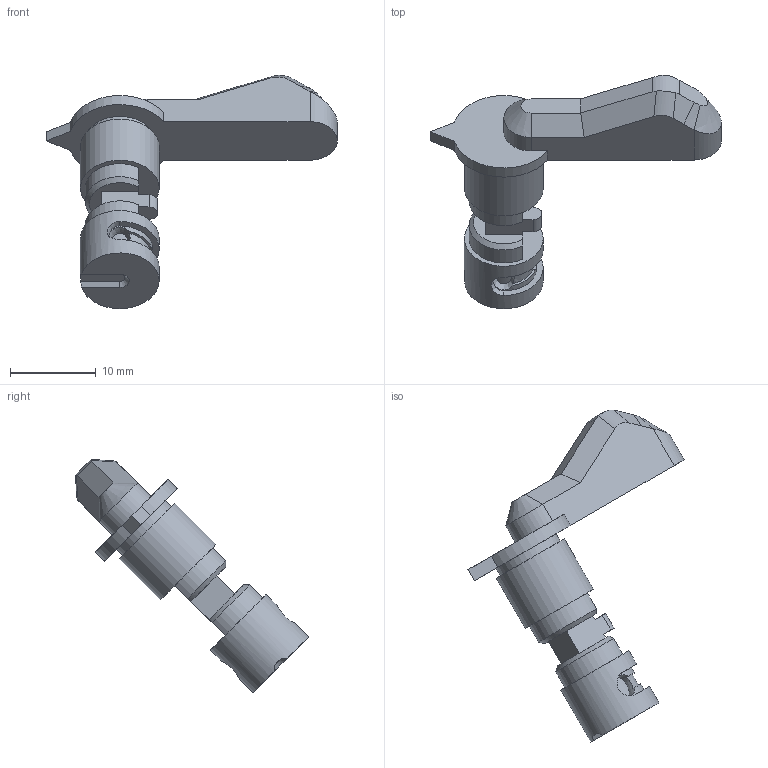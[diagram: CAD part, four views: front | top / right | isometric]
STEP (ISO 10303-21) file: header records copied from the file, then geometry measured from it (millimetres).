
FILE_DESCRIPTION(/* description */ (''),/* implementation_level */ '2;1');
FILE_NAME(/* name */ '',/* time_stamp */ '2021-12-08T23:02:19-05:00',/* author */ (''),/* organization */ (''),/* preprocessor_version */ 'ST-DEVELOPER v18.1',/* originating_system */ 'Autodesk Inventor 2022',/* authorisation */ '');
FILE_SCHEMA (('AUTOMOTIVE_DESIGN { 1 0 10303 214 3 1 1 }'));
Length unit declared in the file: inch
Products named in the file (1): ChoosyBoogleSelectorEnhanced
Bounding box: 33.94 x 27.24 x 27.24 mm (x, y, z)
Volume: 2251.1 mm3; surface area: 1609.7 mm2
Topology: 1 solids, 1 shells, 73 faces, 191 edges, 124 vertices
Faces by surface type: plane 37, cylinder 24, bspline 8, cone 4
Full cylindrical faces by diameter (mm): 8.1 x1, 9.2 x2
Entity records: 2895 total; most frequent: CARTESIAN_POINT 1078, ORIENTED_EDGE 382, DIRECTION 341, EDGE_CURVE 191, VERTEX_POINT 124, AXIS2_PLACEMENT_3D 124, LINE 93, VECTOR 93
